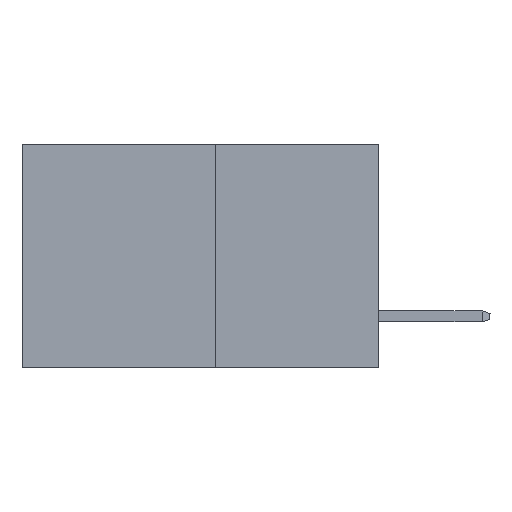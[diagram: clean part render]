
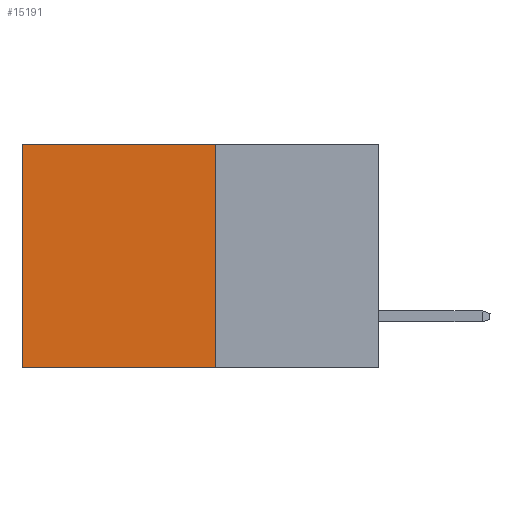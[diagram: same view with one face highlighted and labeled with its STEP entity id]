
A CAD part, left-side view. The second image highlights one B-rep face of the part: STEP entity #15191.
In plain terms, the highlighted planar face has unit normal (-1, 0, 0).
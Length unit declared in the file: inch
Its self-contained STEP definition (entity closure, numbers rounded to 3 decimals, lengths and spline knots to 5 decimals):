
#208 = CARTESIAN_POINT ( 'NONE',  ( 0.277, 0.27, 0. ) ) ;
#559 = VECTOR ( 'NONE', #2471, 39.37008 ) ;
#1137 = CARTESIAN_POINT ( 'NONE',  ( 0.277, 0.59, -0.37 ) ) ;
#1383 = DIRECTION ( 'NONE',  ( 0., 1., 0. ) ) ;
#1465 = EDGE_CURVE ( 'NONE', #31558, #31530, #20584, .T. ) ;
#1529 = VERTEX_POINT ( 'NONE', #208 ) ;
#2352 = ORIENTED_EDGE ( 'NONE', *, *, #29142, .F. ) ;
#2471 = DIRECTION ( 'NONE',  ( 0., 0., -1. ) ) ;
#2579 = CARTESIAN_POINT ( 'NONE',  ( 0.277, 0.27, -0.37 ) ) ;
#2801 = VECTOR ( 'NONE', #12181, 39.37008 ) ;
#2839 = ORIENTED_EDGE ( 'NONE', *, *, #9735, .F. ) ;
#3118 = LINE ( 'NONE', #31548, #15684 ) ;
#4060 = FACE_OUTER_BOUND ( 'NONE', #20322, .T. ) ;
#5109 = DIRECTION ( 'NONE',  ( 1., 0., 0. ) ) ;
#5836 = VERTEX_POINT ( 'NONE', #16135 ) ;
#8330 = VECTOR ( 'NONE', #9794, 39.37008 ) ;
#9735 = EDGE_CURVE ( 'NONE', #1529, #5836, #9937, .T. ) ;
#9794 = DIRECTION ( 'NONE',  ( 0., 0., -1. ) ) ;
#9937 = LINE ( 'NONE', #11557, #8330 ) ;
#11557 = CARTESIAN_POINT ( 'NONE',  ( 0.277, 0.27, -0.37 ) ) ;
#12181 = DIRECTION ( 'NONE',  ( 0., 1., 0. ) ) ;
#15077 = PLANE ( 'NONE',  #20603 ) ;
#15191 = ADVANCED_FACE ( 'NONE', ( #4060 ), #15077, .F. ) ;
#15684 = VECTOR ( 'NONE', #1383, 39.37008 ) ;
#15730 = CARTESIAN_POINT ( 'NONE',  ( 0.277, 0.59, -0.37 ) ) ;
#16135 = CARTESIAN_POINT ( 'NONE',  ( 0.277, 0.27, -0.37 ) ) ;
#17743 = LINE ( 'NONE', #32465, #2801 ) ;
#18279 = CARTESIAN_POINT ( 'NONE',  ( 0.277, 0.59, 0. ) ) ;
#18814 = ORIENTED_EDGE ( 'NONE', *, *, #1465, .T. ) ;
#20322 = EDGE_LOOP ( 'NONE', ( #18814, #2352, #2839, #29762 ) ) ;
#20584 = LINE ( 'NONE', #1137, #559 ) ;
#20603 = AXIS2_PLACEMENT_3D ( 'NONE', #2579, #5109, #22694 ) ;
#22345 = EDGE_CURVE ( 'NONE', #1529, #31558, #17743, .T. ) ;
#22694 = DIRECTION ( 'NONE',  ( 0., 0., -1. ) ) ;
#29142 = EDGE_CURVE ( 'NONE', #5836, #31530, #3118, .T. ) ;
#29762 = ORIENTED_EDGE ( 'NONE', *, *, #22345, .T. ) ;
#31530 = VERTEX_POINT ( 'NONE', #15730 ) ;
#31548 = CARTESIAN_POINT ( 'NONE',  ( 0.277, 0.27, -0.37 ) ) ;
#31558 = VERTEX_POINT ( 'NONE', #18279 ) ;
#32465 = CARTESIAN_POINT ( 'NONE',  ( 0.277, 0.27, 0. ) ) ;
